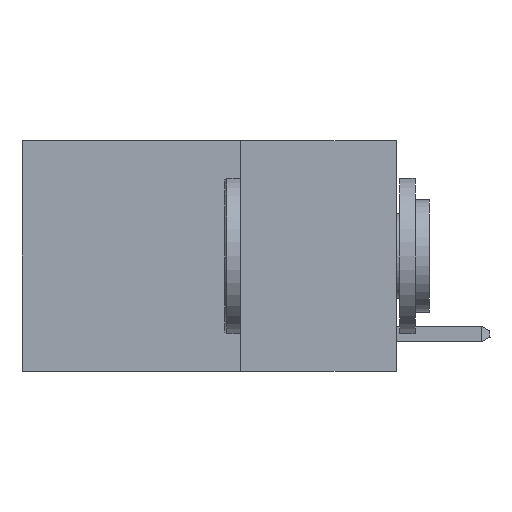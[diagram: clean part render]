
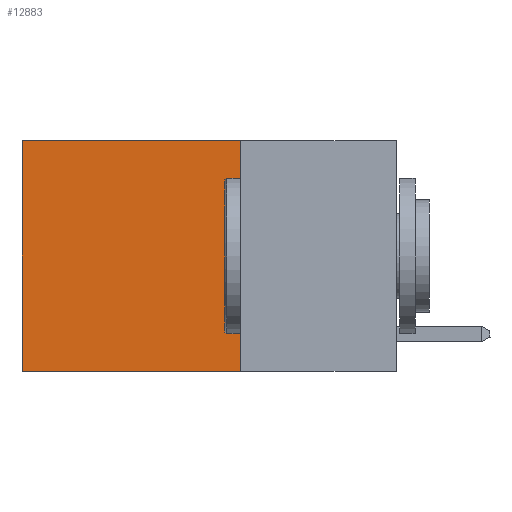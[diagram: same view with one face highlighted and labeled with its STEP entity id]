
A CAD part, left-side view. The second image highlights one B-rep face of the part: STEP entity #12883.
In plain terms, the highlighted planar face has unit normal (-1, 0, 0).
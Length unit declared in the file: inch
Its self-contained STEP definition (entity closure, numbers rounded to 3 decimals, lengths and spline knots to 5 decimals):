
#1555 = ORIENTED_EDGE ( 'NONE', *, *, #7733, .F. ) ;
#1675 = CARTESIAN_POINT ( 'NONE',  ( 0.2625, 0.25, 0. ) ) ;
#2068 = EDGE_CURVE ( 'NONE', #9861, #16983, #9489, .T. ) ;
#2539 = EDGE_LOOP ( 'NONE', ( #26682, #9857, #1555, #12556 ) ) ;
#3163 = CARTESIAN_POINT ( 'NONE',  ( 0.2625, 0.6, -0.37 ) ) ;
#3177 = EDGE_CURVE ( 'NONE', #25089, #16983, #11423, .T. ) ;
#3835 = VECTOR ( 'NONE', #19495, 39.37008 ) ;
#3908 = VERTEX_POINT ( 'NONE', #20786 ) ;
#5090 = DIRECTION ( 'NONE',  ( 1., 0., 0. ) ) ;
#5837 = DIRECTION ( 'NONE',  ( 0., 0., -1. ) ) ;
#6766 = EDGE_CURVE ( 'NONE', #3908, #25089, #24496, .T. ) ;
#6771 = FACE_OUTER_BOUND ( 'NONE', #2539, .T. ) ;
#7212 = AXIS2_PLACEMENT_3D ( 'NONE', #23883, #5090, #19829 ) ;
#7733 = EDGE_CURVE ( 'NONE', #3908, #9861, #12062, .T. ) ;
#9489 = LINE ( 'NONE', #21656, #3835 ) ;
#9857 = ORIENTED_EDGE ( 'NONE', *, *, #2068, .F. ) ;
#9861 = VERTEX_POINT ( 'NONE', #23881 ) ;
#9981 = CARTESIAN_POINT ( 'NONE',  ( 0.2625, 0.6, 0. ) ) ;
#11423 = LINE ( 'NONE', #18474, #26066 ) ;
#12062 = LINE ( 'NONE', #15759, #22493 ) ;
#12556 = ORIENTED_EDGE ( 'NONE', *, *, #6766, .T. ) ;
#12883 = ADVANCED_FACE ( 'NONE', ( #6771 ), #17724, .F. ) ;
#13431 = VECTOR ( 'NONE', #16535, 39.37008 ) ;
#15759 = CARTESIAN_POINT ( 'NONE',  ( 0.2625, 0.25, 0. ) ) ;
#16535 = DIRECTION ( 'NONE',  ( 0., 1., 0. ) ) ;
#16983 = VERTEX_POINT ( 'NONE', #3163 ) ;
#17724 = PLANE ( 'NONE',  #7212 ) ;
#17857 = DIRECTION ( 'NONE',  ( 0., 0., -1. ) ) ;
#18474 = CARTESIAN_POINT ( 'NONE',  ( 0.2625, 0.6, 0. ) ) ;
#19495 = DIRECTION ( 'NONE',  ( 0., 1., 0. ) ) ;
#19829 = DIRECTION ( 'NONE',  ( 0., 0., -1. ) ) ;
#20786 = CARTESIAN_POINT ( 'NONE',  ( 0.2625, 0.25, 0. ) ) ;
#21656 = CARTESIAN_POINT ( 'NONE',  ( 0.2625, 0.25, -0.37 ) ) ;
#22493 = VECTOR ( 'NONE', #17857, 39.37008 ) ;
#23881 = CARTESIAN_POINT ( 'NONE',  ( 0.2625, 0.25, -0.37 ) ) ;
#23883 = CARTESIAN_POINT ( 'NONE',  ( 0.2625, 0.25, 0. ) ) ;
#24496 = LINE ( 'NONE', #1675, #13431 ) ;
#25089 = VERTEX_POINT ( 'NONE', #9981 ) ;
#26066 = VECTOR ( 'NONE', #5837, 39.37008 ) ;
#26682 = ORIENTED_EDGE ( 'NONE', *, *, #3177, .T. ) ;
